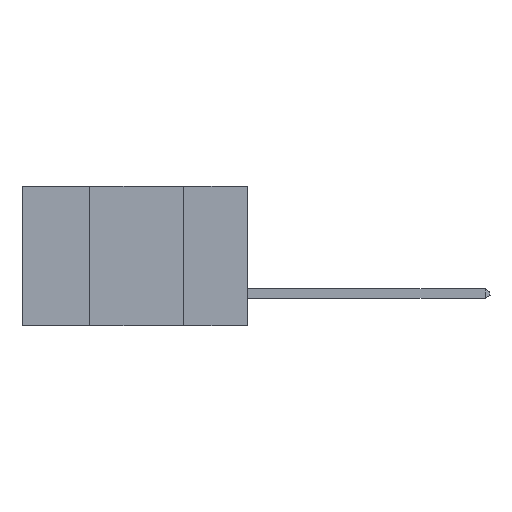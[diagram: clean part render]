
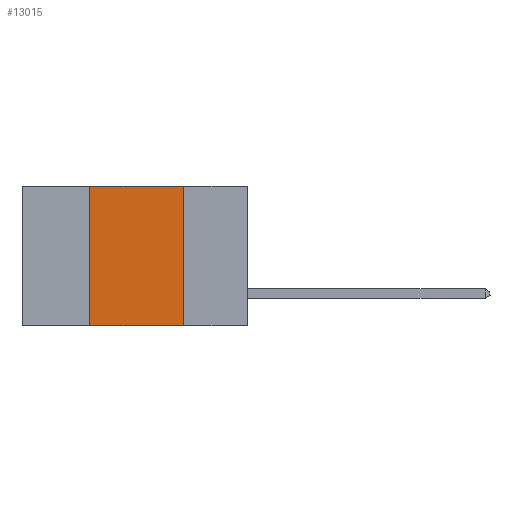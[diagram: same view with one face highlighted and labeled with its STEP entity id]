
A CAD part, left-side view. The second image highlights one B-rep face of the part: STEP entity #13015.
In plain terms, the highlighted planar face has unit normal (-1, 0, 0).
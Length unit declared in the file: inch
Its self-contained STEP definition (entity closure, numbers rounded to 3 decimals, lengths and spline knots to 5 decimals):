
#1329 = DIRECTION ( 'NONE',  ( 0., 0., -1. ) ) ;
#1638 = DIRECTION ( 'NONE',  ( 0., -1., 0. ) ) ;
#2600 = ORIENTED_EDGE ( 'NONE', *, *, #8273, .F. ) ;
#2717 = CARTESIAN_POINT ( 'NONE',  ( 0., 0.17, 0. ) ) ;
#2850 = LINE ( 'NONE', #2717, #11385 ) ;
#3700 = AXIS2_PLACEMENT_3D ( 'NONE', #11733, #8732, #11599 ) ;
#3898 = CARTESIAN_POINT ( 'NONE',  ( 0., 0.17, 0. ) ) ;
#4068 = CARTESIAN_POINT ( 'NONE',  ( 0., 0.42, -0.37 ) ) ;
#4331 = VERTEX_POINT ( 'NONE', #4068 ) ;
#4667 = CARTESIAN_POINT ( 'NONE',  ( 0., 0.6, -0.37 ) ) ;
#5219 = ORIENTED_EDGE ( 'NONE', *, *, #11915, .F. ) ;
#5402 = LINE ( 'NONE', #4667, #18824 ) ;
#5776 = VERTEX_POINT ( 'NONE', #14840 ) ;
#6270 = EDGE_LOOP ( 'NONE', ( #5219, #14956, #2600, #16208 ) ) ;
#7021 = EDGE_CURVE ( 'NONE', #17760, #12803, #7181, .T. ) ;
#7181 = LINE ( 'NONE', #16371, #13180 ) ;
#8273 = EDGE_CURVE ( 'NONE', #4331, #17760, #15476, .T. ) ;
#8732 = DIRECTION ( 'NONE',  ( 1., 0., 0. ) ) ;
#8831 = FACE_OUTER_BOUND ( 'NONE', #6270, .T. ) ;
#9248 = DIRECTION ( 'NONE',  ( 0., 0., 1. ) ) ;
#9841 = EDGE_CURVE ( 'NONE', #4331, #5776, #5402, .T. ) ;
#10127 = PLANE ( 'NONE',  #3700 ) ;
#10628 = DIRECTION ( 'NONE',  ( 0., -1., 0. ) ) ;
#11385 = VECTOR ( 'NONE', #1329, 39.37008 ) ;
#11599 = DIRECTION ( 'NONE',  ( 0., 0., -1. ) ) ;
#11733 = CARTESIAN_POINT ( 'NONE',  ( 0., 0.6, 0. ) ) ;
#11915 = EDGE_CURVE ( 'NONE', #12803, #5776, #2850, .T. ) ;
#12659 = VECTOR ( 'NONE', #9248, 39.37008 ) ;
#12803 = VERTEX_POINT ( 'NONE', #3898 ) ;
#13015 = ADVANCED_FACE ( 'NONE', ( #8831 ), #10127, .F. ) ;
#13180 = VECTOR ( 'NONE', #1638, 39.37008 ) ;
#13472 = CARTESIAN_POINT ( 'NONE',  ( 0., 0.42, 0. ) ) ;
#14736 = CARTESIAN_POINT ( 'NONE',  ( 0., 0.42, 0. ) ) ;
#14840 = CARTESIAN_POINT ( 'NONE',  ( 0., 0.17, -0.37 ) ) ;
#14956 = ORIENTED_EDGE ( 'NONE', *, *, #7021, .F. ) ;
#15476 = LINE ( 'NONE', #13472, #12659 ) ;
#16208 = ORIENTED_EDGE ( 'NONE', *, *, #9841, .T. ) ;
#16371 = CARTESIAN_POINT ( 'NONE',  ( 0., 0.6, 0. ) ) ;
#17760 = VERTEX_POINT ( 'NONE', #14736 ) ;
#18824 = VECTOR ( 'NONE', #10628, 39.37008 ) ;
